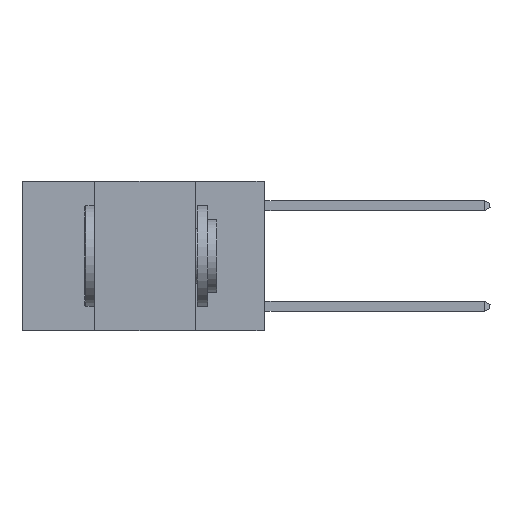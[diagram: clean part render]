
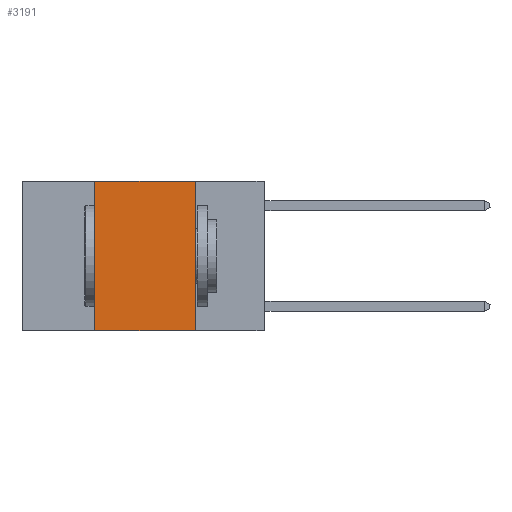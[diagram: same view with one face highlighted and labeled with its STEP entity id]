
A CAD part, left-side view. The second image highlights one B-rep face of the part: STEP entity #3191.
In plain terms, the highlighted planar face has unit normal (-1, 0, 0).
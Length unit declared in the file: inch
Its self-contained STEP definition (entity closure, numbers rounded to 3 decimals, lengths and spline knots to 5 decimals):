
#2047 = EDGE_CURVE ( 'NONE', #5829, #5838, #8779, .T. ) ;
#2250 = EDGE_CURVE ( 'NONE', #7571, #5829, #15320, .T. ) ;
#3191 = ADVANCED_FACE ( 'NONE', ( #13788 ), #9416, .F. ) ;
#4299 = CARTESIAN_POINT ( 'NONE',  ( 0., 0.6, 0. ) ) ;
#4588 = CARTESIAN_POINT ( 'NONE',  ( 0., 0.42, -0.37 ) ) ;
#5043 = VECTOR ( 'NONE', #7251, 39.37008 ) ;
#5095 = AXIS2_PLACEMENT_3D ( 'NONE', #14740, #12770, #15440 ) ;
#5445 = VERTEX_POINT ( 'NONE', #4588 ) ;
#5829 = VERTEX_POINT ( 'NONE', #15886 ) ;
#5838 = VERTEX_POINT ( 'NONE', #9341 ) ;
#6176 = EDGE_CURVE ( 'NONE', #5445, #7571, #17165, .T. ) ;
#6409 = ORIENTED_EDGE ( 'NONE', *, *, #8805, .T. ) ;
#7251 = DIRECTION ( 'NONE',  ( 0., -1., 0. ) ) ;
#7571 = VERTEX_POINT ( 'NONE', #14536 ) ;
#7650 = ORIENTED_EDGE ( 'NONE', *, *, #6176, .F. ) ;
#7851 = VECTOR ( 'NONE', #8618, 39.37008 ) ;
#8618 = DIRECTION ( 'NONE',  ( 0., 0., -1. ) ) ;
#8779 = LINE ( 'NONE', #12538, #7851 ) ;
#8805 = EDGE_CURVE ( 'NONE', #5445, #5838, #13226, .T. ) ;
#9143 = DIRECTION ( 'NONE',  ( 0., 0., 1. ) ) ;
#9341 = CARTESIAN_POINT ( 'NONE',  ( 0., 0.17, -0.37 ) ) ;
#9416 = PLANE ( 'NONE',  #5095 ) ;
#9607 = ORIENTED_EDGE ( 'NONE', *, *, #2250, .F. ) ;
#10538 = CARTESIAN_POINT ( 'NONE',  ( 0., 0.6, -0.37 ) ) ;
#10566 = CARTESIAN_POINT ( 'NONE',  ( 0., 0.42, 0. ) ) ;
#11696 = VECTOR ( 'NONE', #9143, 39.37008 ) ;
#12538 = CARTESIAN_POINT ( 'NONE',  ( 0., 0.17, 0. ) ) ;
#12770 = DIRECTION ( 'NONE',  ( 1., 0., 0. ) ) ;
#13226 = LINE ( 'NONE', #10538, #16222 ) ;
#13234 = EDGE_LOOP ( 'NONE', ( #13713, #9607, #7650, #6409 ) ) ;
#13713 = ORIENTED_EDGE ( 'NONE', *, *, #2047, .F. ) ;
#13788 = FACE_OUTER_BOUND ( 'NONE', #13234, .T. ) ;
#14536 = CARTESIAN_POINT ( 'NONE',  ( 0., 0.42, 0. ) ) ;
#14740 = CARTESIAN_POINT ( 'NONE',  ( 0., 0.6, 0. ) ) ;
#15320 = LINE ( 'NONE', #4299, #5043 ) ;
#15440 = DIRECTION ( 'NONE',  ( 0., 0., -1. ) ) ;
#15886 = CARTESIAN_POINT ( 'NONE',  ( 0., 0.17, 0. ) ) ;
#16099 = DIRECTION ( 'NONE',  ( 0., -1., 0. ) ) ;
#16222 = VECTOR ( 'NONE', #16099, 39.37008 ) ;
#17165 = LINE ( 'NONE', #10566, #11696 ) ;
